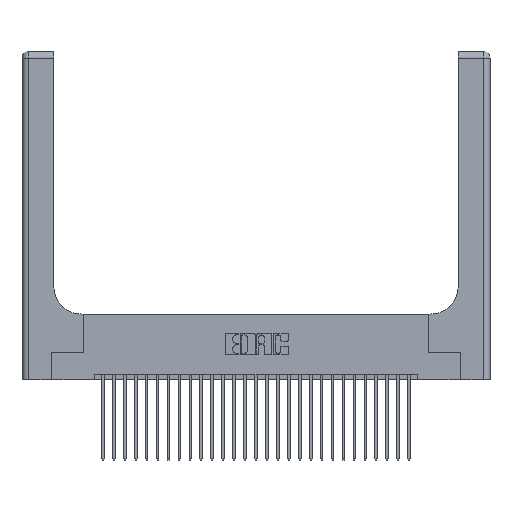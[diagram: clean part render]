
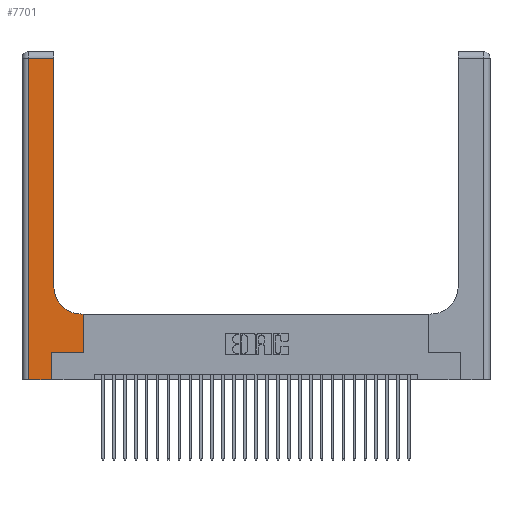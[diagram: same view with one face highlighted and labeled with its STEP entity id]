
A CAD part, top view. The second image highlights one B-rep face of the part: STEP entity #7701.
In plain terms, the highlighted planar face has unit normal (0, 0, 1).
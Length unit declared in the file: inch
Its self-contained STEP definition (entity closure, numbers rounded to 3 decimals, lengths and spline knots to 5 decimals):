
#301 = DIRECTION ( 'NONE',  ( 0., 1., 0. ) ) ;
#1368 = EDGE_CURVE ( 'NONE', #10889, #21811, #5791, .T. ) ;
#1617 = ORIENTED_EDGE ( 'NONE', *, *, #19920, .T. ) ;
#2076 = DIRECTION ( 'NONE',  ( -1., 0., 0. ) ) ;
#2686 = LINE ( 'NONE', #21749, #29641 ) ;
#3785 = ORIENTED_EDGE ( 'NONE', *, *, #22677, .T. ) ;
#4241 = LINE ( 'NONE', #27281, #27908 ) ;
#4500 = DIRECTION ( 'NONE',  ( 0., 1., 0. ) ) ;
#4805 = EDGE_CURVE ( 'NONE', #28958, #13992, #19718, .T. ) ;
#4846 = ORIENTED_EDGE ( 'NONE', *, *, #12921, .T. ) ;
#5124 = VERTEX_POINT ( 'NONE', #23415 ) ;
#5437 = AXIS2_PLACEMENT_3D ( 'NONE', #18004, #20421, #9026 ) ;
#5474 = DIRECTION ( 'NONE',  ( -1., 0., 0. ) ) ;
#5791 = LINE ( 'NONE', #16871, #20829 ) ;
#6577 = CARTESIAN_POINT ( 'NONE',  ( 0., 2.94, 0.37 ) ) ;
#7042 = VERTEX_POINT ( 'NONE', #13164 ) ;
#7056 = LINE ( 'NONE', #27444, #14197 ) ;
#7252 = VERTEX_POINT ( 'NONE', #8763 ) ;
#7371 = LINE ( 'NONE', #18567, #18837 ) ;
#7423 = CARTESIAN_POINT ( 'NONE',  ( 0.269, 0.25, 0.37 ) ) ;
#7701 = ADVANCED_FACE ( 'NONE', ( #20327 ), #14239, .F. ) ;
#8003 = VECTOR ( 'NONE', #301, 39.37008 ) ;
#8320 = ORIENTED_EDGE ( 'NONE', *, *, #14749, .T. ) ;
#8677 = ORIENTED_EDGE ( 'NONE', *, *, #23339, .T. ) ;
#8694 = VERTEX_POINT ( 'NONE', #26540 ) ;
#8763 = CARTESIAN_POINT ( 'NONE',  ( 0.2915, 2.94, 0.37 ) ) ;
#9026 = DIRECTION ( 'NONE',  ( 1., 0., 0. ) ) ;
#10889 = VERTEX_POINT ( 'NONE', #12617 ) ;
#11610 = LINE ( 'NONE', #25524, #8003 ) ;
#11691 = VERTEX_POINT ( 'NONE', #22115 ) ;
#11967 = CARTESIAN_POINT ( 'NONE',  ( 0.5585, 0.25, 0.37 ) ) ;
#12571 = CARTESIAN_POINT ( 'NONE',  ( 0.269, 0.25, 0.37 ) ) ;
#12617 = CARTESIAN_POINT ( 'NONE',  ( 0.5585, 0.6, 0.37 ) ) ;
#12921 = EDGE_CURVE ( 'NONE', #21811, #8694, #21097, .T. ) ;
#13164 = CARTESIAN_POINT ( 'NONE',  ( 0.06, 0., 0.37 ) ) ;
#13208 = ORIENTED_EDGE ( 'NONE', *, *, #23874, .T. ) ;
#13855 = DIRECTION ( 'NONE',  ( 0., 1., 0. ) ) ;
#13992 = VERTEX_POINT ( 'NONE', #11967 ) ;
#14197 = VECTOR ( 'NONE', #4500, 39.37008 ) ;
#14239 = PLANE ( 'NONE',  #27434 ) ;
#14309 = DIRECTION ( 'NONE',  ( 1., 0., 0. ) ) ;
#14320 = VECTOR ( 'NONE', #14309, 39.37008 ) ;
#14448 = CARTESIAN_POINT ( 'NONE',  ( 0., 3., 0.37 ) ) ;
#14749 = EDGE_CURVE ( 'NONE', #7252, #5124, #26000, .T. ) ;
#16871 = CARTESIAN_POINT ( 'NONE',  ( 0.2915, 0.6, 0.37 ) ) ;
#16917 = DIRECTION ( 'NONE',  ( 1., 0., 0. ) ) ;
#16970 = ORIENTED_EDGE ( 'NONE', *, *, #25116, .T. ) ;
#17449 = ORIENTED_EDGE ( 'NONE', *, *, #1368, .T. ) ;
#18004 = CARTESIAN_POINT ( 'NONE',  ( 0.5415, 0.85, 0.37 ) ) ;
#18567 = CARTESIAN_POINT ( 'NONE',  ( 0.5585, 0.25, 0.37 ) ) ;
#18837 = VECTOR ( 'NONE', #13855, 39.37008 ) ;
#19213 = VECTOR ( 'NONE', #2076, 39.37008 ) ;
#19718 = LINE ( 'NONE', #7423, #14320 ) ;
#19920 = EDGE_CURVE ( 'NONE', #11691, #28958, #11610, .T. ) ;
#20327 = FACE_OUTER_BOUND ( 'NONE', #26801, .T. ) ;
#20421 = DIRECTION ( 'NONE',  ( 0., 0., -1. ) ) ;
#20829 = VECTOR ( 'NONE', #23621, 39.37008 ) ;
#21097 = CIRCLE ( 'NONE', #5437, 0.25 ) ;
#21595 = CARTESIAN_POINT ( 'NONE',  ( 0.5415, 0.6, 0.37 ) ) ;
#21749 = CARTESIAN_POINT ( 'NONE',  ( 0., 0., 0.37 ) ) ;
#21811 = VERTEX_POINT ( 'NONE', #21595 ) ;
#22115 = CARTESIAN_POINT ( 'NONE',  ( 0.269, 0., 0.37 ) ) ;
#22677 = EDGE_CURVE ( 'NONE', #5124, #7042, #4241, .T. ) ;
#23339 = EDGE_CURVE ( 'NONE', #8694, #7252, #7056, .T. ) ;
#23415 = CARTESIAN_POINT ( 'NONE',  ( 0.06, 2.94, 0.37 ) ) ;
#23621 = DIRECTION ( 'NONE',  ( -1., 0., 0. ) ) ;
#23874 = EDGE_CURVE ( 'NONE', #13992, #10889, #7371, .T. ) ;
#25083 = DIRECTION ( 'NONE',  ( 0., -1., 0. ) ) ;
#25116 = EDGE_CURVE ( 'NONE', #7042, #11691, #2686, .T. ) ;
#25377 = ORIENTED_EDGE ( 'NONE', *, *, #4805, .T. ) ;
#25524 = CARTESIAN_POINT ( 'NONE',  ( 0.269, 0., 0.37 ) ) ;
#25776 = DIRECTION ( 'NONE',  ( 0., 0., -1. ) ) ;
#26000 = LINE ( 'NONE', #6577, #19213 ) ;
#26540 = CARTESIAN_POINT ( 'NONE',  ( 0.2915, 0.85, 0.37 ) ) ;
#26801 = EDGE_LOOP ( 'NONE', ( #8677, #8320, #3785, #16970, #1617, #25377, #13208, #17449, #4846 ) ) ;
#27281 = CARTESIAN_POINT ( 'NONE',  ( 0.06, 3., 0.37 ) ) ;
#27434 = AXIS2_PLACEMENT_3D ( 'NONE', #14448, #25776, #5474 ) ;
#27444 = CARTESIAN_POINT ( 'NONE',  ( 0.2915, 3., 0.37 ) ) ;
#27908 = VECTOR ( 'NONE', #25083, 39.37008 ) ;
#28958 = VERTEX_POINT ( 'NONE', #12571 ) ;
#29641 = VECTOR ( 'NONE', #16917, 39.37008 ) ;
